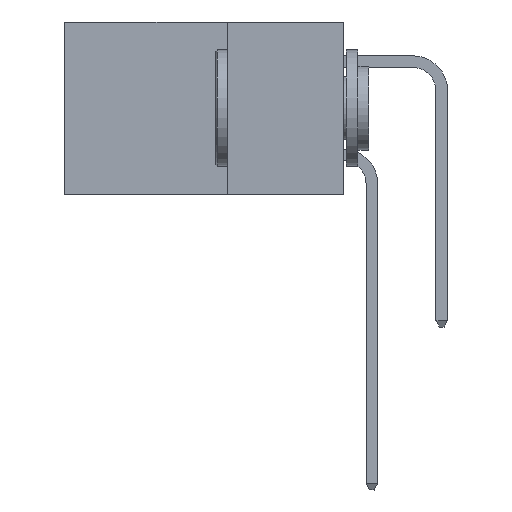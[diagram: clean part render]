
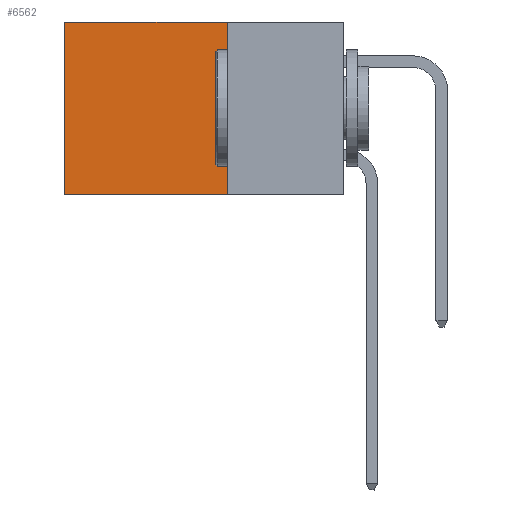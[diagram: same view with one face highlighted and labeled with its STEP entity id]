
A CAD part, left-side view. The second image highlights one B-rep face of the part: STEP entity #6562.
In plain terms, the highlighted planar face has unit normal (-1, 0, 0).
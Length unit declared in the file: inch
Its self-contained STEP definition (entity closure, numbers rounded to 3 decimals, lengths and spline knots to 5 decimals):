
#616 = DIRECTION ( 'NONE',  ( 0., 1., 0. ) ) ;
#832 = DIRECTION ( 'NONE',  ( 0., 0., -1. ) ) ;
#903 = CARTESIAN_POINT ( 'NONE',  ( 0.298, 0.6, 0. ) ) ;
#918 = EDGE_CURVE ( 'NONE', #18928, #8841, #4939, .T. ) ;
#1425 = CARTESIAN_POINT ( 'NONE',  ( 0.298, 0.25, 0. ) ) ;
#1766 = LINE ( 'NONE', #19334, #5475 ) ;
#2041 = CARTESIAN_POINT ( 'NONE',  ( 0.298, 0.6, 0. ) ) ;
#2892 = VERTEX_POINT ( 'NONE', #1425 ) ;
#3122 = CARTESIAN_POINT ( 'NONE',  ( 0.298, 0.25, 0. ) ) ;
#3630 = DIRECTION ( 'NONE',  ( 0., 0., -1. ) ) ;
#3756 = CARTESIAN_POINT ( 'NONE',  ( 0.298, 0.6, -0.37 ) ) ;
#3813 = VERTEX_POINT ( 'NONE', #7919 ) ;
#3928 = EDGE_LOOP ( 'NONE', ( #4926, #12657, #18746, #13323 ) ) ;
#4284 = VECTOR ( 'NONE', #3630, 39.37008 ) ;
#4487 = LINE ( 'NONE', #4811, #11847 ) ;
#4578 = EDGE_CURVE ( 'NONE', #2892, #3813, #12632, .T. ) ;
#4811 = CARTESIAN_POINT ( 'NONE',  ( 0.298, 0.25, 0. ) ) ;
#4926 = ORIENTED_EDGE ( 'NONE', *, *, #918, .T. ) ;
#4939 = LINE ( 'NONE', #903, #9128 ) ;
#5475 = VECTOR ( 'NONE', #616, 39.37008 ) ;
#5734 = EDGE_CURVE ( 'NONE', #2892, #18928, #4487, .T. ) ;
#6246 = DIRECTION ( 'NONE',  ( 0., 1., 0. ) ) ;
#6562 = ADVANCED_FACE ( 'NONE', ( #18559 ), #11864, .F. ) ;
#7919 = CARTESIAN_POINT ( 'NONE',  ( 0.298, 0.25, -0.37 ) ) ;
#8841 = VERTEX_POINT ( 'NONE', #3756 ) ;
#9128 = VECTOR ( 'NONE', #832, 39.37008 ) ;
#10143 = AXIS2_PLACEMENT_3D ( 'NONE', #3122, #18048, #16908 ) ;
#11352 = CARTESIAN_POINT ( 'NONE',  ( 0.298, 0.25, 0. ) ) ;
#11847 = VECTOR ( 'NONE', #6246, 39.37008 ) ;
#11864 = PLANE ( 'NONE',  #10143 ) ;
#12632 = LINE ( 'NONE', #11352, #4284 ) ;
#12657 = ORIENTED_EDGE ( 'NONE', *, *, #15400, .F. ) ;
#13323 = ORIENTED_EDGE ( 'NONE', *, *, #5734, .T. ) ;
#15400 = EDGE_CURVE ( 'NONE', #3813, #8841, #1766, .T. ) ;
#16908 = DIRECTION ( 'NONE',  ( 0., 0., -1. ) ) ;
#18048 = DIRECTION ( 'NONE',  ( 1., 0., 0. ) ) ;
#18559 = FACE_OUTER_BOUND ( 'NONE', #3928, .T. ) ;
#18746 = ORIENTED_EDGE ( 'NONE', *, *, #4578, .F. ) ;
#18928 = VERTEX_POINT ( 'NONE', #2041 ) ;
#19334 = CARTESIAN_POINT ( 'NONE',  ( 0.298, 0.25, -0.37 ) ) ;
